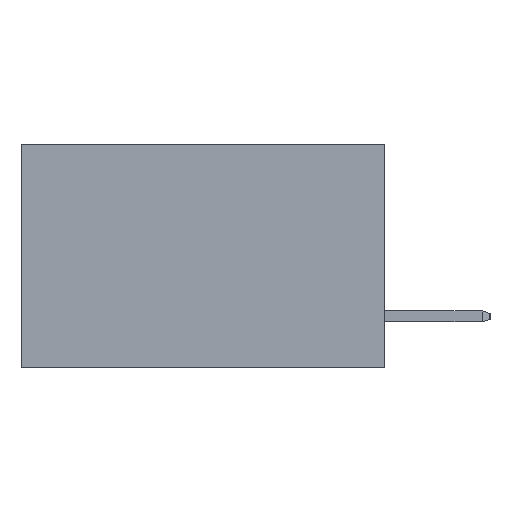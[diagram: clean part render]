
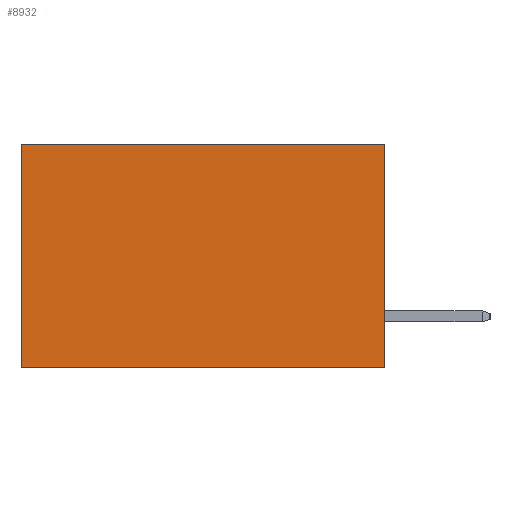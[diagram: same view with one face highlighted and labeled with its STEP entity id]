
A CAD part, left-side view. The second image highlights one B-rep face of the part: STEP entity #8932.
In plain terms, the highlighted planar face has unit normal (-1, 0, 0).
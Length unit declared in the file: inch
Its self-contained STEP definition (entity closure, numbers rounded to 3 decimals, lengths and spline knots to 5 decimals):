
#81 = LINE ( 'NONE', #964, #4250 ) ;
#721 = VERTEX_POINT ( 'NONE', #18957 ) ;
#732 = DIRECTION ( 'NONE',  ( 0., 1., 0. ) ) ;
#964 = CARTESIAN_POINT ( 'NONE',  ( 0.2615, 0.6, -0.37 ) ) ;
#2140 = VECTOR ( 'NONE', #732, 39.37008 ) ;
#2437 = EDGE_CURVE ( 'NONE', #13530, #15891, #3828, .T. ) ;
#3421 = CARTESIAN_POINT ( 'NONE',  ( 0.2615, 0., -0.37 ) ) ;
#3828 = LINE ( 'NONE', #3421, #11879 ) ;
#4250 = VECTOR ( 'NONE', #12281, 39.37008 ) ;
#4741 = ORIENTED_EDGE ( 'NONE', *, *, #5359, .T. ) ;
#4856 = CARTESIAN_POINT ( 'NONE',  ( 0.2615, 0., -0.37 ) ) ;
#5079 = FACE_OUTER_BOUND ( 'NONE', #5248, .T. ) ;
#5165 = VECTOR ( 'NONE', #16551, 39.37008 ) ;
#5216 = EDGE_CURVE ( 'NONE', #15891, #721, #6196, .T. ) ;
#5248 = EDGE_LOOP ( 'NONE', ( #4741, #18002, #14581, #9106 ) ) ;
#5359 = EDGE_CURVE ( 'NONE', #16768, #721, #81, .T. ) ;
#5805 = AXIS2_PLACEMENT_3D ( 'NONE', #15275, #14744, #14718 ) ;
#6196 = LINE ( 'NONE', #4856, #2140 ) ;
#6824 = EDGE_CURVE ( 'NONE', #13530, #16768, #13247, .T. ) ;
#8932 = ADVANCED_FACE ( 'NONE', ( #5079 ), #14888, .F. ) ;
#9106 = ORIENTED_EDGE ( 'NONE', *, *, #6824, .T. ) ;
#11879 = VECTOR ( 'NONE', #13147, 39.37008 ) ;
#12281 = DIRECTION ( 'NONE',  ( 0., 0., -1. ) ) ;
#12644 = CARTESIAN_POINT ( 'NONE',  ( 0.2615, 0., 0. ) ) ;
#13147 = DIRECTION ( 'NONE',  ( 0., 0., -1. ) ) ;
#13247 = LINE ( 'NONE', #16647, #5165 ) ;
#13530 = VERTEX_POINT ( 'NONE', #12644 ) ;
#14581 = ORIENTED_EDGE ( 'NONE', *, *, #2437, .F. ) ;
#14718 = DIRECTION ( 'NONE',  ( 0., 0., -1. ) ) ;
#14744 = DIRECTION ( 'NONE',  ( 1., 0., 0. ) ) ;
#14888 = PLANE ( 'NONE',  #5805 ) ;
#15160 = CARTESIAN_POINT ( 'NONE',  ( 0.2615, 0., -0.37 ) ) ;
#15275 = CARTESIAN_POINT ( 'NONE',  ( 0.2615, 0., -0.37 ) ) ;
#15590 = CARTESIAN_POINT ( 'NONE',  ( 0.2615, 0.6, 0. ) ) ;
#15891 = VERTEX_POINT ( 'NONE', #15160 ) ;
#16551 = DIRECTION ( 'NONE',  ( 0., 1., 0. ) ) ;
#16647 = CARTESIAN_POINT ( 'NONE',  ( 0.2615, 0., 0. ) ) ;
#16768 = VERTEX_POINT ( 'NONE', #15590 ) ;
#18002 = ORIENTED_EDGE ( 'NONE', *, *, #5216, .F. ) ;
#18957 = CARTESIAN_POINT ( 'NONE',  ( 0.2615, 0.6, -0.37 ) ) ;
